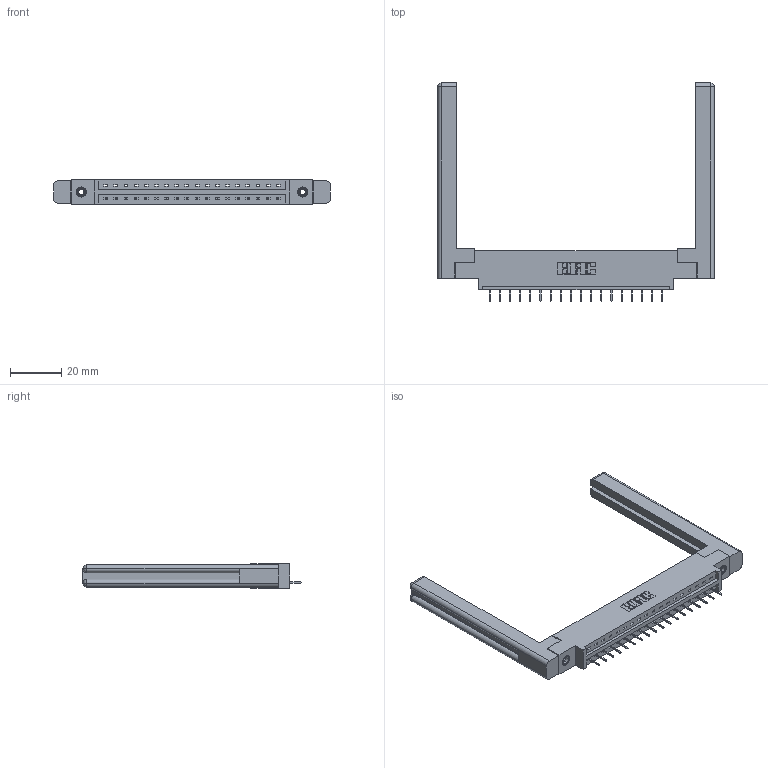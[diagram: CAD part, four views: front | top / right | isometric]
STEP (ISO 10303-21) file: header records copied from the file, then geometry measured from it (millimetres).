
FILE_DESCRIPTION (( 'STEP AP203' ), '1' );
FILE_NAME ('387-018-524-658.STEP', '2019-10-02T20:13:03', ( '' ), ( '' ), 'SwSTEP 2.0', 'SolidWorks 2016', '' );
FILE_SCHEMA (( 'CONFIG_CONTROL_DESIGN' ));
Length unit declared in the file: inch
Products named in the file (5): 387-018-524-658; 307-220-058; 345-250-001_345-250-001-102; 345-292-001_345-293-124; 337 Part_0.170 Offset - 0.156 Dia-TI
Assembly tree (23 placements, depth 2):
  387-018-524-658
    337 Part_0.170 Offset - 0.156 Dia-TI
    345-292-001_345-293-124  x18
    345-250-001_345-250-001-102  x2
    307-220-058  x2
Bounding box: 107.95 x 85.1 x 9.4 mm (x, y, z)
Volume: 17892.8 mm3; surface area: 16014.7 mm2
Topology: 23 solids, 23 shells, 1448 faces, 4133 edges, 2670 vertices
Faces by surface type: plane 1094, cylinder 330, cone 12, torus 12
Entity records: 19324 total; most frequent: CARTESIAN_POINT 3363, ORIENTED_EDGE 3256, DIRECTION 2900, EDGE_CURVE 1628, LINE 1456, VECTOR 1456, VERTEX_POINT 1074, AXIS2_PLACEMENT_3D 722
